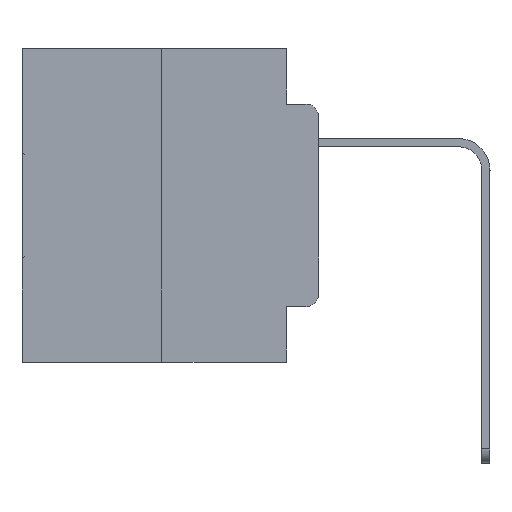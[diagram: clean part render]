
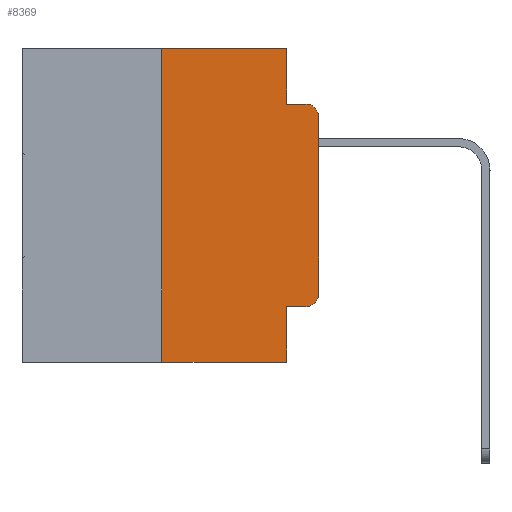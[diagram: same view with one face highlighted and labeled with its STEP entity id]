
A CAD part, left-side view. The second image highlights one B-rep face of the part: STEP entity #8369.
In plain terms, the highlighted planar face has unit normal (-1, 0, 0).
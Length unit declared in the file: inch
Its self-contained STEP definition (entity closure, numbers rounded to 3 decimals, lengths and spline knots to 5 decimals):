
#720 = EDGE_CURVE ( 'NONE', #20253, #25473, #1515, .T. ) ;
#1515 = LINE ( 'NONE', #28035, #25053 ) ;
#2045 = VERTEX_POINT ( 'NONE', #6097 ) ;
#2685 = DIRECTION ( 'NONE',  ( 0., 0., -1. ) ) ;
#3091 = CARTESIAN_POINT ( 'NONE',  ( 0., 0.473, -0.5 ) ) ;
#4025 = ORIENTED_EDGE ( 'NONE', *, *, #13335, .T. ) ;
#4072 = CARTESIAN_POINT ( 'NONE',  ( 0., 0.051, 0. ) ) ;
#4390 = DIRECTION ( 'NONE',  ( 0., -1., 0. ) ) ;
#4997 = EDGE_CURVE ( 'NONE', #19839, #2045, #21569, .T. ) ;
#5154 = LINE ( 'NONE', #14689, #24752 ) ;
#5479 = LINE ( 'NONE', #3091, #28948 ) ;
#6097 = CARTESIAN_POINT ( 'NONE',  ( 0., 0., -0.3915 ) ) ;
#6131 = CARTESIAN_POINT ( 'NONE',  ( 0., 0.051, 0. ) ) ;
#6252 = EDGE_CURVE ( 'NONE', #25473, #15460, #7578, .T. ) ;
#6458 = VERTEX_POINT ( 'NONE', #11928 ) ;
#6469 = CARTESIAN_POINT ( 'NONE',  ( 0., 0.051, -0.0885 ) ) ;
#6723 = EDGE_CURVE ( 'NONE', #6458, #23144, #21103, .T. ) ;
#7379 = CARTESIAN_POINT ( 'NONE',  ( 0., 0.02, -0.4115 ) ) ;
#7578 = LINE ( 'NONE', #12097, #24329 ) ;
#8369 = ADVANCED_FACE ( 'NONE', ( #28434 ), #27958, .F. ) ;
#8656 = ORIENTED_EDGE ( 'NONE', *, *, #25349, .F. ) ;
#9053 = ORIENTED_EDGE ( 'NONE', *, *, #6252, .F. ) ;
#9377 = ORIENTED_EDGE ( 'NONE', *, *, #720, .F. ) ;
#10612 = EDGE_CURVE ( 'NONE', #19548, #17402, #17280, .T. ) ;
#11928 = CARTESIAN_POINT ( 'NONE',  ( 0., 0.051, -0.4115 ) ) ;
#12097 = CARTESIAN_POINT ( 'NONE',  ( 0., 0.051, 0. ) ) ;
#12390 = CARTESIAN_POINT ( 'NONE',  ( 0., 0.25, -0.5 ) ) ;
#13244 = VECTOR ( 'NONE', #4390, 39.37008 ) ;
#13335 = EDGE_CURVE ( 'NONE', #6458, #19839, #19257, .T. ) ;
#13459 = ORIENTED_EDGE ( 'NONE', *, *, #21493, .T. ) ;
#14170 = CARTESIAN_POINT ( 'NONE',  ( 0., 0.051, -0.0885 ) ) ;
#14689 = CARTESIAN_POINT ( 'NONE',  ( 0., 0.25, 0. ) ) ;
#15051 = DIRECTION ( 'NONE',  ( 1., 0., 0. ) ) ;
#15432 = AXIS2_PLACEMENT_3D ( 'NONE', #27444, #22927, #20916 ) ;
#15460 = VERTEX_POINT ( 'NONE', #14170 ) ;
#16792 = VECTOR ( 'NONE', #19984, 39.37008 ) ;
#16810 = DIRECTION ( 'NONE',  ( 0., -1., 0. ) ) ;
#17280 = CIRCLE ( 'NONE', #20879, 0.02 ) ;
#17402 = VERTEX_POINT ( 'NONE', #26175 ) ;
#17525 = CARTESIAN_POINT ( 'NONE',  ( 0., 0., 0. ) ) ;
#17893 = ORIENTED_EDGE ( 'NONE', *, *, #10612, .T. ) ;
#18022 = CARTESIAN_POINT ( 'NONE',  ( 0., 0.051, -0.4115 ) ) ;
#18042 = VECTOR ( 'NONE', #26566, 39.37008 ) ;
#18413 = EDGE_CURVE ( 'NONE', #15460, #17402, #29026, .T. ) ;
#18648 = EDGE_LOOP ( 'NONE', ( #24893, #17893, #26769, #9053, #9377, #8656, #13459, #23076, #4025, #24723 ) ) ;
#18742 = DIRECTION ( 'NONE',  ( 0., 0., -1. ) ) ;
#19257 = LINE ( 'NONE', #18022, #13244 ) ;
#19548 = VERTEX_POINT ( 'NONE', #27076 ) ;
#19618 = DIRECTION ( 'NONE',  ( 0., 0., -1. ) ) ;
#19839 = VERTEX_POINT ( 'NONE', #7379 ) ;
#19984 = DIRECTION ( 'NONE',  ( 0., 0., -1. ) ) ;
#19998 = DIRECTION ( 'NONE',  ( 0., -1., 0. ) ) ;
#20253 = VERTEX_POINT ( 'NONE', #29125 ) ;
#20879 = AXIS2_PLACEMENT_3D ( 'NONE', #25651, #28031, #2685 ) ;
#20916 = DIRECTION ( 'NONE',  ( 0., 0., -1. ) ) ;
#21103 = LINE ( 'NONE', #4072, #16792 ) ;
#21346 = CARTESIAN_POINT ( 'NONE',  ( 0., 0.473, 0. ) ) ;
#21493 = EDGE_CURVE ( 'NONE', #29371, #23144, #5479, .T. ) ;
#21569 = CIRCLE ( 'NONE', #15432, 0.02 ) ;
#22351 = LINE ( 'NONE', #17525, #18042 ) ;
#22679 = VECTOR ( 'NONE', #19998, 39.37008 ) ;
#22927 = DIRECTION ( 'NONE',  ( -1., 0., 0. ) ) ;
#23076 = ORIENTED_EDGE ( 'NONE', *, *, #6723, .F. ) ;
#23144 = VERTEX_POINT ( 'NONE', #27186 ) ;
#23916 = DIRECTION ( 'NONE',  ( 0., -1., 0. ) ) ;
#24329 = VECTOR ( 'NONE', #18742, 39.37008 ) ;
#24489 = EDGE_CURVE ( 'NONE', #2045, #19548, #22351, .T. ) ;
#24723 = ORIENTED_EDGE ( 'NONE', *, *, #4997, .T. ) ;
#24752 = VECTOR ( 'NONE', #27590, 39.37008 ) ;
#24893 = ORIENTED_EDGE ( 'NONE', *, *, #24489, .T. ) ;
#25053 = VECTOR ( 'NONE', #16810, 39.37008 ) ;
#25349 = EDGE_CURVE ( 'NONE', #29371, #20253, #5154, .T. ) ;
#25473 = VERTEX_POINT ( 'NONE', #6131 ) ;
#25651 = CARTESIAN_POINT ( 'NONE',  ( 0., 0.02, -0.1085 ) ) ;
#26175 = CARTESIAN_POINT ( 'NONE',  ( 0., 0.02, -0.0885 ) ) ;
#26566 = DIRECTION ( 'NONE',  ( 0., 0., 1. ) ) ;
#26737 = AXIS2_PLACEMENT_3D ( 'NONE', #21346, #15051, #19618 ) ;
#26769 = ORIENTED_EDGE ( 'NONE', *, *, #18413, .F. ) ;
#27076 = CARTESIAN_POINT ( 'NONE',  ( 0., 0., -0.1085 ) ) ;
#27186 = CARTESIAN_POINT ( 'NONE',  ( 0., 0.051, -0.5 ) ) ;
#27444 = CARTESIAN_POINT ( 'NONE',  ( 0., 0.02, -0.3915 ) ) ;
#27590 = DIRECTION ( 'NONE',  ( 0., 0., 1. ) ) ;
#27958 = PLANE ( 'NONE',  #26737 ) ;
#28031 = DIRECTION ( 'NONE',  ( -1., 0., 0. ) ) ;
#28035 = CARTESIAN_POINT ( 'NONE',  ( 0., 0.473, 0. ) ) ;
#28434 = FACE_OUTER_BOUND ( 'NONE', #18648, .T. ) ;
#28948 = VECTOR ( 'NONE', #23916, 39.37008 ) ;
#29026 = LINE ( 'NONE', #6469, #22679 ) ;
#29125 = CARTESIAN_POINT ( 'NONE',  ( 0., 0.25, 0. ) ) ;
#29371 = VERTEX_POINT ( 'NONE', #12390 ) ;
